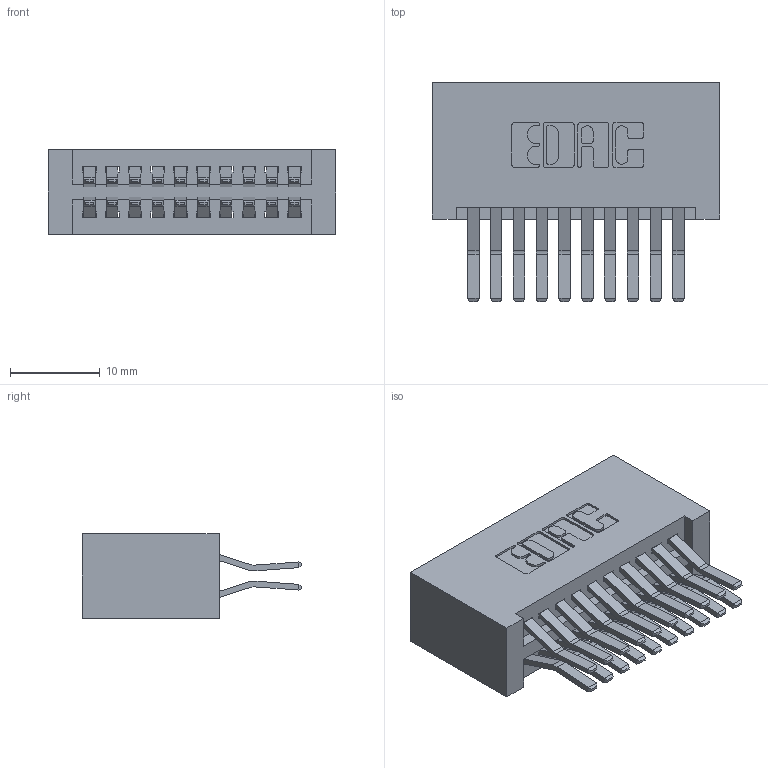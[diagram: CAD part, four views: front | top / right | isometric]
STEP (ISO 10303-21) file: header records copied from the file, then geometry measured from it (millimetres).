
FILE_DESCRIPTION (( 'STEP AP203' ), '1' );
FILE_NAME ('395-020-560-201.STEP', '2019-10-15T22:14:26', ( '' ), ( '' ), 'SwSTEP 2.0', 'SolidWorks 2016', '' );
FILE_SCHEMA (( 'CONFIG_CONTROL_DESIGN' ));
Length unit declared in the file: inch
Products named in the file (3): 345 Part_No Mounting Lugs; 345-292-001_560 Tail; 395-020-560-201
Assembly tree (21 placements, depth 2):
  395-020-560-201
    345 Part_No Mounting Lugs
    345-292-001_560 Tail  x20
Bounding box: 32 x 24.45 x 9.4 mm (x, y, z)
Volume: 3558.9 mm3; surface area: 5281.3 mm2
Topology: 21 solids, 21 shells, 1158 faces, 3417 edges, 2250 vertices
Faces by surface type: plane 736, cylinder 422
Entity records: 11965 total; most frequent: CARTESIAN_POINT 2036, ORIENTED_EDGE 1970, DIRECTION 1833, EDGE_CURVE 985, LINE 817, VECTOR 817, VERTEX_POINT 654, AXIS2_PLACEMENT_3D 508
